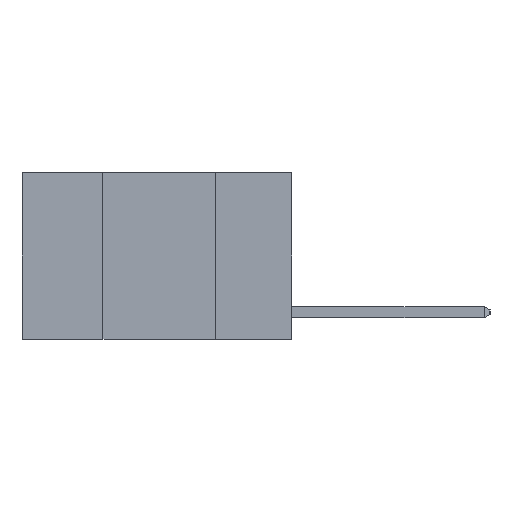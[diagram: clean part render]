
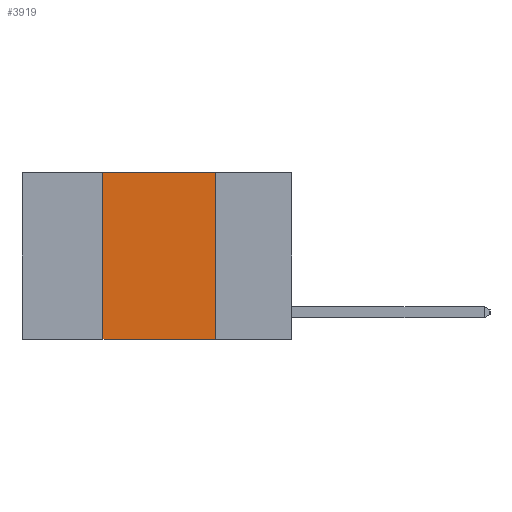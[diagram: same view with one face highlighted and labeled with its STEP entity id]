
A CAD part, left-side view. The second image highlights one B-rep face of the part: STEP entity #3919.
In plain terms, the highlighted planar face has unit normal (-1, 0, 0).
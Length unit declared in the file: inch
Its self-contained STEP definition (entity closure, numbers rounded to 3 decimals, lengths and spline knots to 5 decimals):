
#419 = DIRECTION ( 'NONE',  ( 0., -1., 0. ) ) ;
#480 = CARTESIAN_POINT ( 'NONE',  ( 0., 0.6, 0. ) ) ;
#550 = CARTESIAN_POINT ( 'NONE',  ( 0., 0.17, 0. ) ) ;
#623 = DIRECTION ( 'NONE',  ( 0., 0., -1. ) ) ;
#679 = ORIENTED_EDGE ( 'NONE', *, *, #6910, .F. ) ;
#718 = VERTEX_POINT ( 'NONE', #1627 ) ;
#880 = ORIENTED_EDGE ( 'NONE', *, *, #3136, .F. ) ;
#1019 = LINE ( 'NONE', #6396, #1213 ) ;
#1049 = LINE ( 'NONE', #6366, #7857 ) ;
#1173 = EDGE_CURVE ( 'NONE', #6307, #6315, #1049, .T. ) ;
#1213 = VECTOR ( 'NONE', #7003, 39.37008 ) ;
#1331 = EDGE_LOOP ( 'NONE', ( #3957, #679, #880, #4364 ) ) ;
#1493 = EDGE_CURVE ( 'NONE', #3814, #6315, #5668, .T. ) ;
#1627 = CARTESIAN_POINT ( 'NONE',  ( 0., 0.42, 0. ) ) ;
#2211 = VECTOR ( 'NONE', #5250, 39.37008 ) ;
#2438 = VECTOR ( 'NONE', #5030, 39.37008 ) ;
#3136 = EDGE_CURVE ( 'NONE', #6307, #718, #1019, .T. ) ;
#3205 = CARTESIAN_POINT ( 'NONE',  ( 0., 0.6, 0. ) ) ;
#3814 = VERTEX_POINT ( 'NONE', #7456 ) ;
#3919 = ADVANCED_FACE ( 'NONE', ( #6130 ), #5736, .F. ) ;
#3957 = ORIENTED_EDGE ( 'NONE', *, *, #1493, .F. ) ;
#4364 = ORIENTED_EDGE ( 'NONE', *, *, #1173, .T. ) ;
#4538 = DIRECTION ( 'NONE',  ( 1., 0., 0. ) ) ;
#5030 = DIRECTION ( 'NONE',  ( 0., -1., 0. ) ) ;
#5250 = DIRECTION ( 'NONE',  ( 0., 0., -1. ) ) ;
#5493 = CARTESIAN_POINT ( 'NONE',  ( 0., 0.42, -0.37 ) ) ;
#5668 = LINE ( 'NONE', #550, #2211 ) ;
#5736 = PLANE ( 'NONE',  #7251 ) ;
#6130 = FACE_OUTER_BOUND ( 'NONE', #1331, .T. ) ;
#6307 = VERTEX_POINT ( 'NONE', #5493 ) ;
#6315 = VERTEX_POINT ( 'NONE', #7434 ) ;
#6366 = CARTESIAN_POINT ( 'NONE',  ( 0., 0.6, -0.37 ) ) ;
#6396 = CARTESIAN_POINT ( 'NONE',  ( 0., 0.42, 0. ) ) ;
#6910 = EDGE_CURVE ( 'NONE', #718, #3814, #7415, .T. ) ;
#7003 = DIRECTION ( 'NONE',  ( 0., 0., 1. ) ) ;
#7251 = AXIS2_PLACEMENT_3D ( 'NONE', #3205, #4538, #623 ) ;
#7415 = LINE ( 'NONE', #480, #2438 ) ;
#7434 = CARTESIAN_POINT ( 'NONE',  ( 0., 0.17, -0.37 ) ) ;
#7456 = CARTESIAN_POINT ( 'NONE',  ( 0., 0.17, 0. ) ) ;
#7857 = VECTOR ( 'NONE', #419, 39.37008 ) ;
